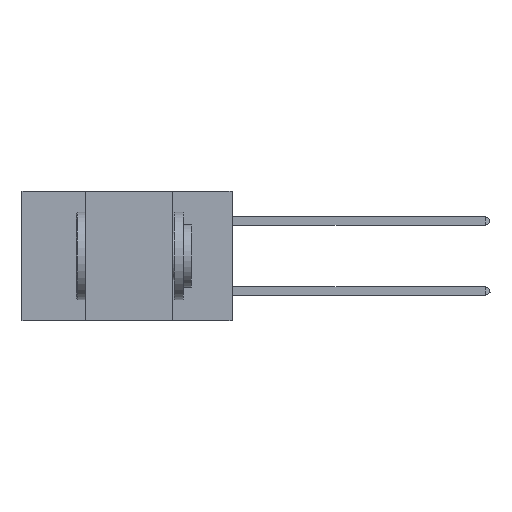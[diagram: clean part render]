
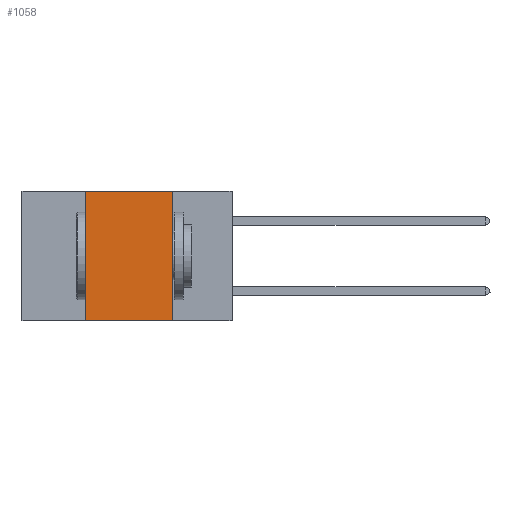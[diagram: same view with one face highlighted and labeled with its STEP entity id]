
A CAD part, left-side view. The second image highlights one B-rep face of the part: STEP entity #1058.
In plain terms, the highlighted planar face has unit normal (-1, 0, 0).
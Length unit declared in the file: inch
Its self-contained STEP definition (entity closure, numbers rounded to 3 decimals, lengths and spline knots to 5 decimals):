
#57 = DIRECTION ( 'NONE',  ( 0., 0., -1. ) ) ;
#108 = DIRECTION ( 'NONE',  ( 1., 0., 0. ) ) ;
#1050 = EDGE_CURVE ( 'NONE', #6915, #4910, #8272, .T. ) ;
#1058 = ADVANCED_FACE ( 'NONE', ( #1269 ), #8928, .F. ) ;
#1062 = ORIENTED_EDGE ( 'NONE', *, *, #5448, .F. ) ;
#1269 = FACE_OUTER_BOUND ( 'NONE', #8284, .T. ) ;
#2733 = CARTESIAN_POINT ( 'NONE',  ( 0., 0.6, 0. ) ) ;
#2842 = ORIENTED_EDGE ( 'NONE', *, *, #3809, .F. ) ;
#3192 = VERTEX_POINT ( 'NONE', #10285 ) ;
#3743 = ORIENTED_EDGE ( 'NONE', *, *, #1050, .T. ) ;
#3809 = EDGE_CURVE ( 'NONE', #3192, #7747, #10937, .T. ) ;
#4571 = DIRECTION ( 'NONE',  ( 0., -1., 0. ) ) ;
#4801 = LINE ( 'NONE', #5366, #8703 ) ;
#4910 = VERTEX_POINT ( 'NONE', #6906 ) ;
#5366 = CARTESIAN_POINT ( 'NONE',  ( 0., 0.17, 0. ) ) ;
#5448 = EDGE_CURVE ( 'NONE', #7747, #4910, #4801, .T. ) ;
#6423 = CARTESIAN_POINT ( 'NONE',  ( 0., 0.42, 0. ) ) ;
#6854 = VECTOR ( 'NONE', #4571, 39.37008 ) ;
#6906 = CARTESIAN_POINT ( 'NONE',  ( 0., 0.17, -0.37 ) ) ;
#6915 = VERTEX_POINT ( 'NONE', #8364 ) ;
#7747 = VERTEX_POINT ( 'NONE', #11321 ) ;
#8076 = CARTESIAN_POINT ( 'NONE',  ( 0., 0.6, -0.37 ) ) ;
#8097 = CARTESIAN_POINT ( 'NONE',  ( 0., 0.6, 0. ) ) ;
#8272 = LINE ( 'NONE', #8076, #6854 ) ;
#8284 = EDGE_LOOP ( 'NONE', ( #1062, #2842, #9218, #3743 ) ) ;
#8364 = CARTESIAN_POINT ( 'NONE',  ( 0., 0.42, -0.37 ) ) ;
#8605 = VECTOR ( 'NONE', #9821, 39.37008 ) ;
#8703 = VECTOR ( 'NONE', #57, 39.37008 ) ;
#8928 = PLANE ( 'NONE',  #10429 ) ;
#9218 = ORIENTED_EDGE ( 'NONE', *, *, #9515, .F. ) ;
#9515 = EDGE_CURVE ( 'NONE', #6915, #3192, #9559, .T. ) ;
#9559 = LINE ( 'NONE', #6423, #11320 ) ;
#9821 = DIRECTION ( 'NONE',  ( 0., -1., 0. ) ) ;
#10094 = DIRECTION ( 'NONE',  ( 0., 0., 1. ) ) ;
#10285 = CARTESIAN_POINT ( 'NONE',  ( 0., 0.42, 0. ) ) ;
#10429 = AXIS2_PLACEMENT_3D ( 'NONE', #2733, #108, #10672 ) ;
#10672 = DIRECTION ( 'NONE',  ( 0., 0., -1. ) ) ;
#10937 = LINE ( 'NONE', #8097, #8605 ) ;
#11320 = VECTOR ( 'NONE', #10094, 39.37008 ) ;
#11321 = CARTESIAN_POINT ( 'NONE',  ( 0., 0.17, 0. ) ) ;
